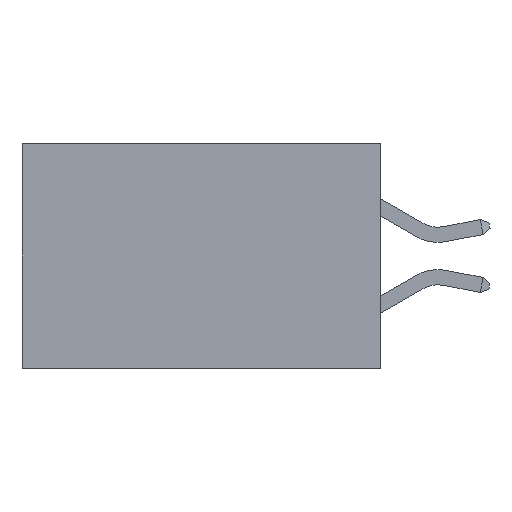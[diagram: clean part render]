
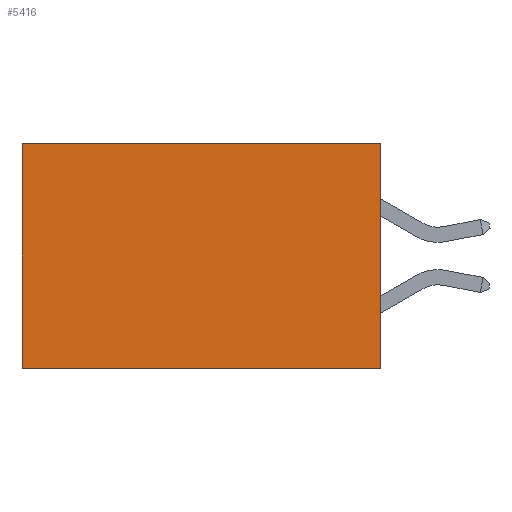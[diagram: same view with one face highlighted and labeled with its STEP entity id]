
A CAD part, left-side view. The second image highlights one B-rep face of the part: STEP entity #5416.
In plain terms, the highlighted planar face has unit normal (-1, 0, 0).
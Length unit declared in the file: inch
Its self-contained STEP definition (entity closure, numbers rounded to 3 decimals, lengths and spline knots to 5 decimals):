
#200 = VERTEX_POINT ( 'NONE', #8342 ) ;
#325 = ORIENTED_EDGE ( 'NONE', *, *, #4723, .T. ) ;
#344 = VERTEX_POINT ( 'NONE', #4148 ) ;
#374 = LINE ( 'NONE', #5612, #4049 ) ;
#1193 = VERTEX_POINT ( 'NONE', #1711 ) ;
#1506 = CARTESIAN_POINT ( 'NONE',  ( 0.277, 0., 0. ) ) ;
#1665 = DIRECTION ( 'NONE',  ( 0., 0., -1. ) ) ;
#1711 = CARTESIAN_POINT ( 'NONE',  ( 0.277, 0., -0.37 ) ) ;
#1748 = DIRECTION ( 'NONE',  ( 0., 0., -1. ) ) ;
#2120 = LINE ( 'NONE', #3981, #9322 ) ;
#2379 = EDGE_CURVE ( 'NONE', #1193, #200, #2120, .T. ) ;
#3467 = CARTESIAN_POINT ( 'NONE',  ( 0.277, 0., -0.37 ) ) ;
#3514 = CARTESIAN_POINT ( 'NONE',  ( 0.277, 0., 0. ) ) ;
#3598 = FACE_OUTER_BOUND ( 'NONE', #8821, .T. ) ;
#3609 = LINE ( 'NONE', #5666, #7087 ) ;
#3981 = CARTESIAN_POINT ( 'NONE',  ( 0.277, 0., -0.37 ) ) ;
#4049 = VECTOR ( 'NONE', #5632, 39.37008 ) ;
#4055 = VECTOR ( 'NONE', #5764, 39.37008 ) ;
#4148 = CARTESIAN_POINT ( 'NONE',  ( 0.277, 0.59, 0. ) ) ;
#4674 = ORIENTED_EDGE ( 'NONE', *, *, #5240, .T. ) ;
#4723 = EDGE_CURVE ( 'NONE', #7364, #344, #6110, .T. ) ;
#4802 = EDGE_CURVE ( 'NONE', #7364, #1193, #3609, .T. ) ;
#5240 = EDGE_CURVE ( 'NONE', #344, #200, #374, .T. ) ;
#5416 = ADVANCED_FACE ( 'NONE', ( #3598 ), #6972, .F. ) ;
#5424 = AXIS2_PLACEMENT_3D ( 'NONE', #3467, #7611, #1665 ) ;
#5612 = CARTESIAN_POINT ( 'NONE',  ( 0.277, 0.59, -0.37 ) ) ;
#5632 = DIRECTION ( 'NONE',  ( 0., 0., -1. ) ) ;
#5666 = CARTESIAN_POINT ( 'NONE',  ( 0.277, 0., -0.37 ) ) ;
#5764 = DIRECTION ( 'NONE',  ( 0., 1., 0. ) ) ;
#5982 = ORIENTED_EDGE ( 'NONE', *, *, #2379, .F. ) ;
#6110 = LINE ( 'NONE', #1506, #4055 ) ;
#6972 = PLANE ( 'NONE',  #5424 ) ;
#7087 = VECTOR ( 'NONE', #1748, 39.37008 ) ;
#7364 = VERTEX_POINT ( 'NONE', #3514 ) ;
#7568 = DIRECTION ( 'NONE',  ( 0., 1., 0. ) ) ;
#7611 = DIRECTION ( 'NONE',  ( 1., 0., 0. ) ) ;
#7839 = ORIENTED_EDGE ( 'NONE', *, *, #4802, .F. ) ;
#8342 = CARTESIAN_POINT ( 'NONE',  ( 0.277, 0.59, -0.37 ) ) ;
#8821 = EDGE_LOOP ( 'NONE', ( #4674, #5982, #7839, #325 ) ) ;
#9322 = VECTOR ( 'NONE', #7568, 39.37008 ) ;
